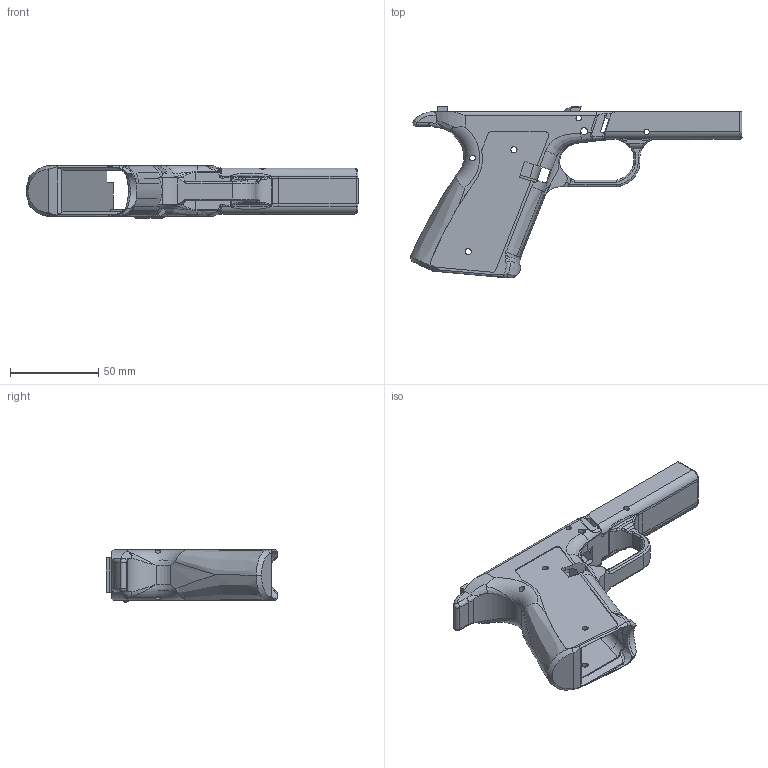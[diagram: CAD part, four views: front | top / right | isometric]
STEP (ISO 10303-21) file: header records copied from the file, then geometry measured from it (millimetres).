
FILE_DESCRIPTION(/* description */ (''),/* implementation_level */ '2;1');
FILE_NAME(/* name */ 'G19Eleven Frame.step',/* time_stamp */ '2022-05-10T10:22:48-06:00',/* author */ (''),/* organization */ (''),/* preprocessor_version */ 'ST-DEVELOPER v18.1',/* originating_system */ 'Autodesk Translation Framework v10.14.0.1471',/* authorisation */ '');
FILE_SCHEMA (('AUTOMOTIVE_DESIGN { 1 0 10303 214 3 1 1 }'));
Products named in the file (1): G1911
Bounding box: 188.07 x 97 x 29.84 mm (x, y, z)
Volume: 83653.3 mm3; surface area: 44304.1 mm2
Topology: 1 solids, 1 shells, 634 faces, 1825 edges, 1167 vertices
Faces by surface type: plane 208, bspline 181, cylinder 174, torus 54, sphere 12, cone 5
Full cylindrical faces by diameter (mm): 2 x1, 3 x4, 3.2 x2, 3.5 x4, 4 x2
Entity records: 37628 total; most frequent: CARTESIAN_POINT 22123, ORIENTED_EDGE 3632, DIRECTION 2751, EDGE_CURVE 1816, VERTEX_POINT 1166, AXIS2_PLACEMENT_3D 1000, LINE 751, VECTOR 751
